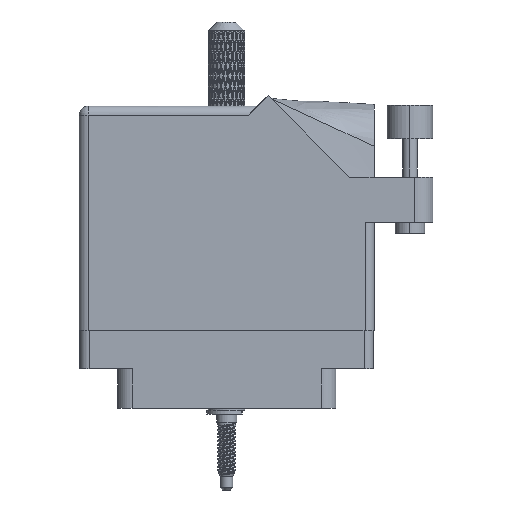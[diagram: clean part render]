
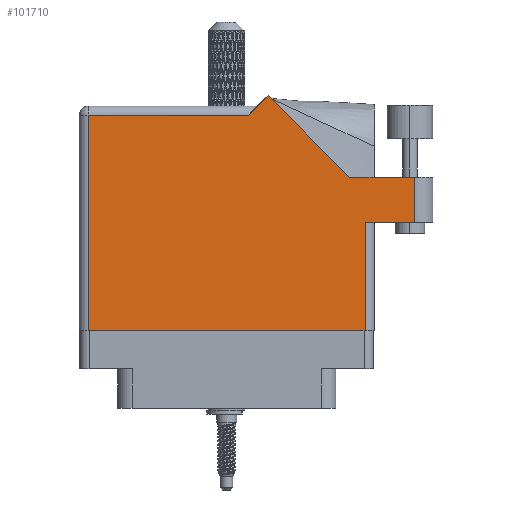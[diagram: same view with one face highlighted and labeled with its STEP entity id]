
A CAD part, front view. The second image highlights one B-rep face of the part: STEP entity #101710.
In plain terms, the highlighted face is planar.
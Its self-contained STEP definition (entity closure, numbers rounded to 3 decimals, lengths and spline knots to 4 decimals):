
#422 = DIRECTION ( 'NONE',  ( 0., 1., 0. ) ) ;
#1951 = EDGE_CURVE ( 'NONE', #4083, #47065, #36733, .T. ) ;
#3111 = LINE ( 'NONE', #100183, #65188 ) ;
#3196 = DIRECTION ( 'NONE',  ( 1., 0., 0. ) ) ;
#4083 = VERTEX_POINT ( 'NONE', #36111 ) ;
#5649 = DIRECTION ( 'NONE',  ( -0.707, -0.707, 0. ) ) ;
#5899 = EDGE_CURVE ( 'NONE', #71713, #24562, #41649, .T. ) ;
#9816 = ORIENTED_EDGE ( 'NONE', *, *, #1951, .T. ) ;
#10035 = EDGE_CURVE ( 'NONE', #18714, #20968, #78969, .T. ) ;
#10797 = EDGE_CURVE ( 'NONE', #74991, #71713, #30857, .T. ) ;
#11041 = CARTESIAN_POINT ( 'NONE',  ( 0.062, 1.468, 0. ) ) ;
#11478 = VERTEX_POINT ( 'NONE', #11041 ) ;
#12280 = LINE ( 'NONE', #40844, #65398 ) ;
#13104 = CARTESIAN_POINT ( 'NONE',  ( 1.217, 1.53, 0. ) ) ;
#17698 = DIRECTION ( 'NONE',  ( -0.707, 0.707, 0. ) ) ;
#18714 = VERTEX_POINT ( 'NONE', #46828 ) ;
#19483 = EDGE_CURVE ( 'NONE', #91927, #74991, #21831, .T. ) ;
#20583 = ORIENTED_EDGE ( 'NONE', *, *, #19483, .T. ) ;
#20968 = VERTEX_POINT ( 'NONE', #59227 ) ;
#21831 = LINE ( 'NONE', #73702, #69965 ) ;
#24562 = VERTEX_POINT ( 'NONE', #59526 ) ;
#28367 = DIRECTION ( 'NONE',  ( -1., 0., 0. ) ) ;
#28668 = CARTESIAN_POINT ( 'NONE',  ( 1.2877, 1.6007, 0. ) ) ;
#30857 = LINE ( 'NONE', #58040, #62442 ) ;
#31876 = CARTESIAN_POINT ( 'NONE',  ( 2.285, 0.737, 0. ) ) ;
#33442 = DIRECTION ( 'NONE',  ( -1., 0., 0. ) ) ;
#36111 = CARTESIAN_POINT ( 'NONE',  ( 1.948, 0.737, 0. ) ) ;
#36165 = EDGE_CURVE ( 'NONE', #47065, #91927, #3111, .T. ) ;
#36733 = LINE ( 'NONE', #98072, #49399 ) ;
#40604 = CARTESIAN_POINT ( 'NONE',  ( 2.285, 1.044, 0. ) ) ;
#40844 = CARTESIAN_POINT ( 'NONE',  ( 1.948, 0.737, 0. ) ) ;
#40944 = EDGE_CURVE ( 'NONE', #24562, #11478, #71918, .T. ) ;
#41297 = AXIS2_PLACEMENT_3D ( 'NONE', #48036, #64969, #72027 ) ;
#41649 = LINE ( 'NONE', #13104, #83430 ) ;
#46828 = CARTESIAN_POINT ( 'NONE',  ( 0.062, 0., 0. ) ) ;
#47065 = VERTEX_POINT ( 'NONE', #31876 ) ;
#48036 = CARTESIAN_POINT ( 'NONE',  ( 0., 1.53, 0. ) ) ;
#48146 = CARTESIAN_POINT ( 'NONE',  ( 0.062, 0., 0. ) ) ;
#49399 = VECTOR ( 'NONE', #57733, 39.3701 ) ;
#52475 = DIRECTION ( 'NONE',  ( 0., 1., 0. ) ) ;
#55365 = FACE_OUTER_BOUND ( 'NONE', #58476, .T. ) ;
#55760 = EDGE_CURVE ( 'NONE', #20968, #4083, #12280, .T. ) ;
#57733 = DIRECTION ( 'NONE',  ( 1., 0., 0. ) ) ;
#58040 = CARTESIAN_POINT ( 'NONE',  ( 1.8444, 1.044, 0. ) ) ;
#58476 = EDGE_LOOP ( 'NONE', ( #9816, #64915, #20583, #94341, #80395, #79337, #85571, #87591, #91195 ) ) ;
#59227 = CARTESIAN_POINT ( 'NONE',  ( 1.948, 0., 0. ) ) ;
#59526 = CARTESIAN_POINT ( 'NONE',  ( 1.155, 1.468, 0. ) ) ;
#62442 = VECTOR ( 'NONE', #17698, 39.3701 ) ;
#64893 = EDGE_CURVE ( 'NONE', #11478, #18714, #103361, .T. ) ;
#64915 = ORIENTED_EDGE ( 'NONE', *, *, #36165, .T. ) ;
#64969 = DIRECTION ( 'NONE',  ( 0., 0., -1. ) ) ;
#65188 = VECTOR ( 'NONE', #52475, 39.3701 ) ;
#65398 = VECTOR ( 'NONE', #422, 39.3701 ) ;
#69965 = VECTOR ( 'NONE', #33442, 39.3701 ) ;
#71089 = DIRECTION ( 'NONE',  ( 0., -1., 0. ) ) ;
#71713 = VERTEX_POINT ( 'NONE', #28668 ) ;
#71918 = LINE ( 'NONE', #92066, #97225 ) ;
#72027 = DIRECTION ( 'NONE',  ( -1., 0., 0. ) ) ;
#73702 = CARTESIAN_POINT ( 'NONE',  ( 2.41, 1.044, 0. ) ) ;
#74991 = VERTEX_POINT ( 'NONE', #86999 ) ;
#78969 = LINE ( 'NONE', #100864, #91662 ) ;
#79337 = ORIENTED_EDGE ( 'NONE', *, *, #40944, .T. ) ;
#79858 = PLANE ( 'NONE',  #41297 ) ;
#80395 = ORIENTED_EDGE ( 'NONE', *, *, #5899, .T. ) ;
#83144 = VECTOR ( 'NONE', #71089, 39.3701 ) ;
#83430 = VECTOR ( 'NONE', #5649, 39.3701 ) ;
#85571 = ORIENTED_EDGE ( 'NONE', *, *, #64893, .T. ) ;
#86999 = CARTESIAN_POINT ( 'NONE',  ( 1.8444, 1.044, 0. ) ) ;
#87591 = ORIENTED_EDGE ( 'NONE', *, *, #10035, .T. ) ;
#91195 = ORIENTED_EDGE ( 'NONE', *, *, #55760, .T. ) ;
#91662 = VECTOR ( 'NONE', #3196, 39.3701 ) ;
#91927 = VERTEX_POINT ( 'NONE', #40604 ) ;
#92066 = CARTESIAN_POINT ( 'NONE',  ( 0., 1.468, 0. ) ) ;
#94341 = ORIENTED_EDGE ( 'NONE', *, *, #10797, .T. ) ;
#97225 = VECTOR ( 'NONE', #28367, 39.3701 ) ;
#98072 = CARTESIAN_POINT ( 'NONE',  ( 2.01, 0.737, 0. ) ) ;
#100183 = CARTESIAN_POINT ( 'NONE',  ( 2.285, 1.044, 0. ) ) ;
#100864 = CARTESIAN_POINT ( 'NONE',  ( 0., 0., 0. ) ) ;
#101710 = ADVANCED_FACE ( 'NONE', ( #55365 ), #79858, .F. ) ;
#103361 = LINE ( 'NONE', #48146, #83144 ) ;
